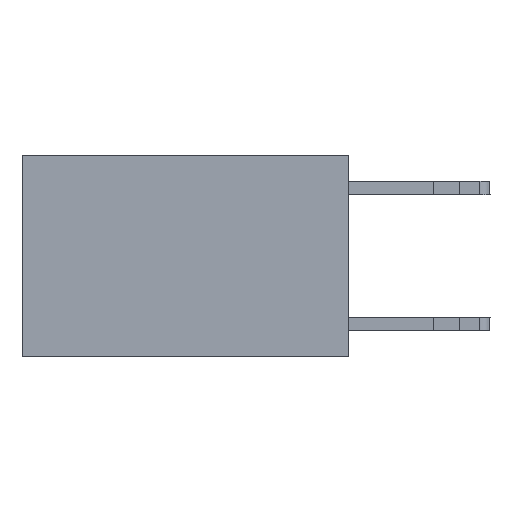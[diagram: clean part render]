
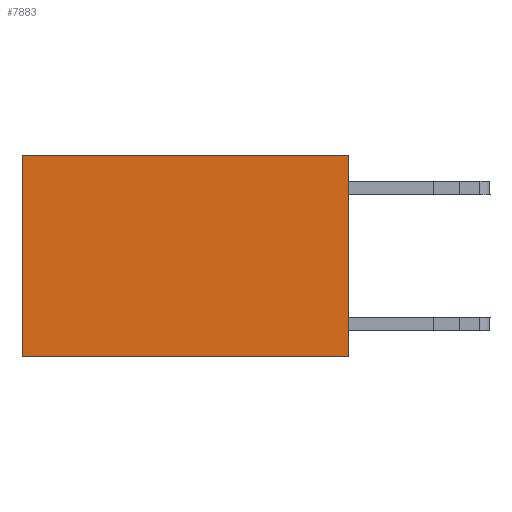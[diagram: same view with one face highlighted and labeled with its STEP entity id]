
A CAD part, left-side view. The second image highlights one B-rep face of the part: STEP entity #7883.
In plain terms, the highlighted planar face has unit normal (-1, 0, 0).
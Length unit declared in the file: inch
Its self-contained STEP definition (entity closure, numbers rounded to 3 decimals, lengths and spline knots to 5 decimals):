
#726 = CARTESIAN_POINT ( 'NONE',  ( 0.2625, 0., -0.37 ) ) ;
#1113 = VERTEX_POINT ( 'NONE', #12017 ) ;
#1914 = VECTOR ( 'NONE', #12644, 39.37008 ) ;
#2364 = CARTESIAN_POINT ( 'NONE',  ( 0.2625, 0., -0.37 ) ) ;
#2391 = VERTEX_POINT ( 'NONE', #3724 ) ;
#2504 = DIRECTION ( 'NONE',  ( 0., 1., 0. ) ) ;
#3100 = VECTOR ( 'NONE', #10428, 39.37008 ) ;
#3441 = ORIENTED_EDGE ( 'NONE', *, *, #10780, .F. ) ;
#3588 = DIRECTION ( 'NONE',  ( 1., 0., 0. ) ) ;
#3606 = LINE ( 'NONE', #8313, #10258 ) ;
#3672 = CARTESIAN_POINT ( 'NONE',  ( 0.2625, 0., 0. ) ) ;
#3724 = CARTESIAN_POINT ( 'NONE',  ( 0.2625, 0.6, -0.37 ) ) ;
#5256 = VERTEX_POINT ( 'NONE', #726 ) ;
#5679 = LINE ( 'NONE', #10598, #1914 ) ;
#6196 = FACE_OUTER_BOUND ( 'NONE', #6520, .T. ) ;
#6388 = EDGE_CURVE ( 'NONE', #1113, #10548, #3606, .T. ) ;
#6520 = EDGE_LOOP ( 'NONE', ( #14737, #9768, #3441, #13907 ) ) ;
#6878 = LINE ( 'NONE', #10276, #3100 ) ;
#7027 = DIRECTION ( 'NONE',  ( 0., 1., 0. ) ) ;
#7883 = ADVANCED_FACE ( 'NONE', ( #6196 ), #10613, .F. ) ;
#8078 = EDGE_CURVE ( 'NONE', #5256, #2391, #10595, .T. ) ;
#8313 = CARTESIAN_POINT ( 'NONE',  ( 0.2625, 0., 0. ) ) ;
#9768 = ORIENTED_EDGE ( 'NONE', *, *, #8078, .F. ) ;
#10258 = VECTOR ( 'NONE', #2504, 39.37008 ) ;
#10276 = CARTESIAN_POINT ( 'NONE',  ( 0.2625, 0., 0. ) ) ;
#10428 = DIRECTION ( 'NONE',  ( 0., 0., -1. ) ) ;
#10548 = VERTEX_POINT ( 'NONE', #11877 ) ;
#10595 = LINE ( 'NONE', #2364, #13008 ) ;
#10598 = CARTESIAN_POINT ( 'NONE',  ( 0.2625, 0.6, 0. ) ) ;
#10613 = PLANE ( 'NONE',  #12780 ) ;
#10780 = EDGE_CURVE ( 'NONE', #1113, #5256, #6878, .T. ) ;
#11249 = EDGE_CURVE ( 'NONE', #10548, #2391, #5679, .T. ) ;
#11877 = CARTESIAN_POINT ( 'NONE',  ( 0.2625, 0.6, 0. ) ) ;
#12017 = CARTESIAN_POINT ( 'NONE',  ( 0.2625, 0., 0. ) ) ;
#12644 = DIRECTION ( 'NONE',  ( 0., 0., -1. ) ) ;
#12780 = AXIS2_PLACEMENT_3D ( 'NONE', #3672, #3588, #14392 ) ;
#13008 = VECTOR ( 'NONE', #7027, 39.37008 ) ;
#13907 = ORIENTED_EDGE ( 'NONE', *, *, #6388, .T. ) ;
#14392 = DIRECTION ( 'NONE',  ( 0., 0., -1. ) ) ;
#14737 = ORIENTED_EDGE ( 'NONE', *, *, #11249, .T. ) ;
